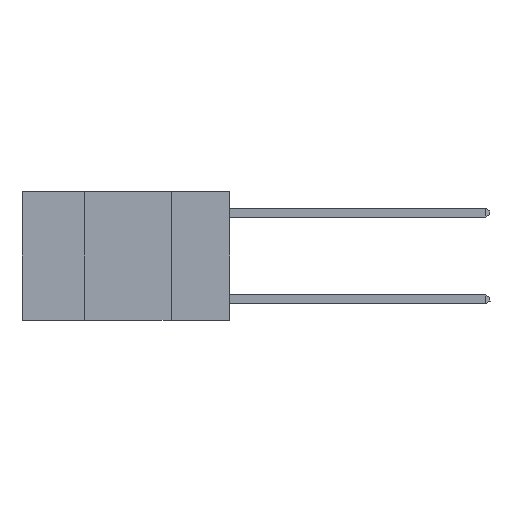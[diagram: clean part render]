
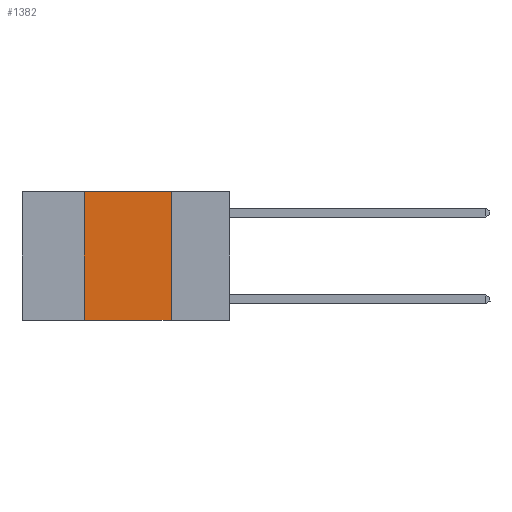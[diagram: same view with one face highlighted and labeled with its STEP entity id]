
A CAD part, left-side view. The second image highlights one B-rep face of the part: STEP entity #1382.
In plain terms, the highlighted planar face has unit normal (-1, 0, 0).
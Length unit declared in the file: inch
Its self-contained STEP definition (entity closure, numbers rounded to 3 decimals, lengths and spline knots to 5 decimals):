
#1094 = EDGE_CURVE ( 'NONE', #22433, #31371, #2621, .T. ) ;
#1205 = DIRECTION ( 'NONE',  ( 0., 0., 1. ) ) ;
#1382 = ADVANCED_FACE ( 'NONE', ( #18732 ), #26361, .F. ) ;
#1783 = CARTESIAN_POINT ( 'NONE',  ( 0., 0.42, 0. ) ) ;
#2621 = LINE ( 'NONE', #4572, #5958 ) ;
#3201 = CARTESIAN_POINT ( 'NONE',  ( 0., 0.42, 0. ) ) ;
#4572 = CARTESIAN_POINT ( 'NONE',  ( 0., 0.6, 0. ) ) ;
#5958 = VECTOR ( 'NONE', #12552, 39.37008 ) ;
#6358 = DIRECTION ( 'NONE',  ( 1., 0., 0. ) ) ;
#6978 = VERTEX_POINT ( 'NONE', #30210 ) ;
#7122 = LINE ( 'NONE', #19647, #14561 ) ;
#8499 = ORIENTED_EDGE ( 'NONE', *, *, #31057, .T. ) ;
#11762 = EDGE_CURVE ( 'NONE', #6978, #22433, #23355, .T. ) ;
#11839 = LINE ( 'NONE', #27133, #15915 ) ;
#12552 = DIRECTION ( 'NONE',  ( 0., -1., 0. ) ) ;
#12689 = EDGE_CURVE ( 'NONE', #31371, #20440, #7122, .T. ) ;
#12924 = AXIS2_PLACEMENT_3D ( 'NONE', #13700, #6358, #26682 ) ;
#13700 = CARTESIAN_POINT ( 'NONE',  ( 0., 0.6, 0. ) ) ;
#14561 = VECTOR ( 'NONE', #17212, 39.37008 ) ;
#15915 = VECTOR ( 'NONE', #22689, 39.37008 ) ;
#17212 = DIRECTION ( 'NONE',  ( 0., 0., -1. ) ) ;
#18732 = FACE_OUTER_BOUND ( 'NONE', #26239, .T. ) ;
#19647 = CARTESIAN_POINT ( 'NONE',  ( 0., 0.17, 0. ) ) ;
#19966 = CARTESIAN_POINT ( 'NONE',  ( 0., 0.17, -0.37 ) ) ;
#20440 = VERTEX_POINT ( 'NONE', #19966 ) ;
#21076 = ORIENTED_EDGE ( 'NONE', *, *, #11762, .F. ) ;
#21860 = ORIENTED_EDGE ( 'NONE', *, *, #1094, .F. ) ;
#22433 = VERTEX_POINT ( 'NONE', #1783 ) ;
#22560 = ORIENTED_EDGE ( 'NONE', *, *, #12689, .F. ) ;
#22689 = DIRECTION ( 'NONE',  ( 0., -1., 0. ) ) ;
#23355 = LINE ( 'NONE', #3201, #26374 ) ;
#26239 = EDGE_LOOP ( 'NONE', ( #22560, #21860, #21076, #8499 ) ) ;
#26361 = PLANE ( 'NONE',  #12924 ) ;
#26374 = VECTOR ( 'NONE', #1205, 39.37008 ) ;
#26682 = DIRECTION ( 'NONE',  ( 0., 0., -1. ) ) ;
#27133 = CARTESIAN_POINT ( 'NONE',  ( 0., 0.6, -0.37 ) ) ;
#30210 = CARTESIAN_POINT ( 'NONE',  ( 0., 0.42, -0.37 ) ) ;
#31012 = CARTESIAN_POINT ( 'NONE',  ( 0., 0.17, 0. ) ) ;
#31057 = EDGE_CURVE ( 'NONE', #6978, #20440, #11839, .T. ) ;
#31371 = VERTEX_POINT ( 'NONE', #31012 ) ;
